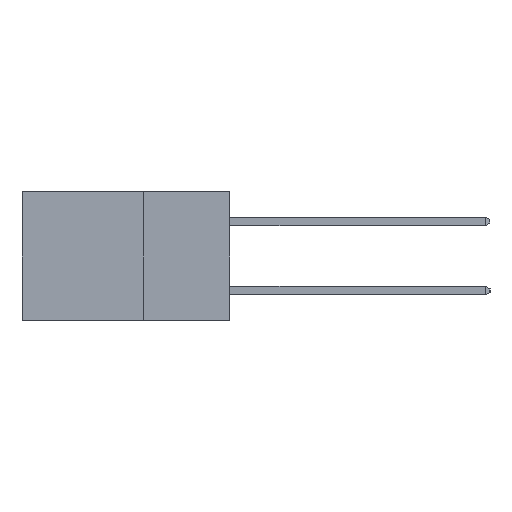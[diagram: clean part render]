
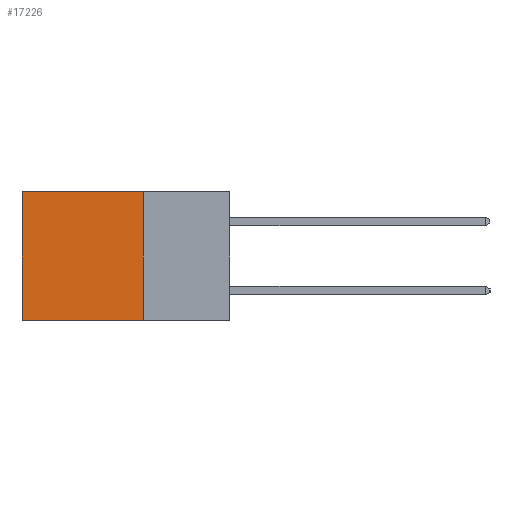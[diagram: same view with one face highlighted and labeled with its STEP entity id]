
A CAD part, left-side view. The second image highlights one B-rep face of the part: STEP entity #17226.
In plain terms, the highlighted planar face has unit normal (-1, 0, 0).
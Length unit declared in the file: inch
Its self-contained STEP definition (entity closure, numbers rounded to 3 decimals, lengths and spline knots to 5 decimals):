
#672 = DIRECTION ( 'NONE',  ( 0., 1., 0. ) ) ;
#773 = DIRECTION ( 'NONE',  ( 0., 0., -1. ) ) ;
#818 = EDGE_CURVE ( 'NONE', #4940, #7298, #14553, .T. ) ;
#1286 = VECTOR ( 'NONE', #13733, 39.37008 ) ;
#2438 = ORIENTED_EDGE ( 'NONE', *, *, #14095, .F. ) ;
#3040 = VECTOR ( 'NONE', #773, 39.37008 ) ;
#3489 = LINE ( 'NONE', #17031, #3040 ) ;
#3998 = VECTOR ( 'NONE', #14031, 39.37008 ) ;
#4031 = PLANE ( 'NONE',  #15061 ) ;
#4034 = CARTESIAN_POINT ( 'NONE',  ( 0.2615, 0.6, -0.37 ) ) ;
#4940 = VERTEX_POINT ( 'NONE', #9038 ) ;
#5357 = CARTESIAN_POINT ( 'NONE',  ( 0.2615, 0.25, -0.37 ) ) ;
#5387 = FACE_OUTER_BOUND ( 'NONE', #13708, .T. ) ;
#5497 = VECTOR ( 'NONE', #672, 39.37008 ) ;
#5991 = CARTESIAN_POINT ( 'NONE',  ( 0.2615, 0.6, 0. ) ) ;
#6362 = VERTEX_POINT ( 'NONE', #5991 ) ;
#6778 = DIRECTION ( 'NONE',  ( 0., 0., -1. ) ) ;
#7200 = ORIENTED_EDGE ( 'NONE', *, *, #818, .F. ) ;
#7298 = VERTEX_POINT ( 'NONE', #4034 ) ;
#7657 = CARTESIAN_POINT ( 'NONE',  ( 0.2615, 0.25, 0. ) ) ;
#8245 = EDGE_CURVE ( 'NONE', #6362, #7298, #3489, .T. ) ;
#9038 = CARTESIAN_POINT ( 'NONE',  ( 0.2615, 0.25, -0.37 ) ) ;
#11220 = LINE ( 'NONE', #12676, #3998 ) ;
#12676 = CARTESIAN_POINT ( 'NONE',  ( 0.2615, 0.25, -0.37 ) ) ;
#13050 = CARTESIAN_POINT ( 'NONE',  ( 0.2615, 0.25, 0. ) ) ;
#13085 = LINE ( 'NONE', #13050, #5497 ) ;
#13708 = EDGE_LOOP ( 'NONE', ( #17576, #7200, #2438, #13997 ) ) ;
#13733 = DIRECTION ( 'NONE',  ( 0., 1., 0. ) ) ;
#13948 = CARTESIAN_POINT ( 'NONE',  ( 0.2615, 0.25, -0.37 ) ) ;
#13997 = ORIENTED_EDGE ( 'NONE', *, *, #14226, .T. ) ;
#14031 = DIRECTION ( 'NONE',  ( 0., 0., -1. ) ) ;
#14095 = EDGE_CURVE ( 'NONE', #15510, #4940, #11220, .T. ) ;
#14226 = EDGE_CURVE ( 'NONE', #15510, #6362, #13085, .T. ) ;
#14553 = LINE ( 'NONE', #13948, #1286 ) ;
#14818 = DIRECTION ( 'NONE',  ( 1., 0., 0. ) ) ;
#15061 = AXIS2_PLACEMENT_3D ( 'NONE', #5357, #14818, #6778 ) ;
#15510 = VERTEX_POINT ( 'NONE', #7657 ) ;
#17031 = CARTESIAN_POINT ( 'NONE',  ( 0.2615, 0.6, -0.37 ) ) ;
#17226 = ADVANCED_FACE ( 'NONE', ( #5387 ), #4031, .F. ) ;
#17576 = ORIENTED_EDGE ( 'NONE', *, *, #8245, .T. ) ;
